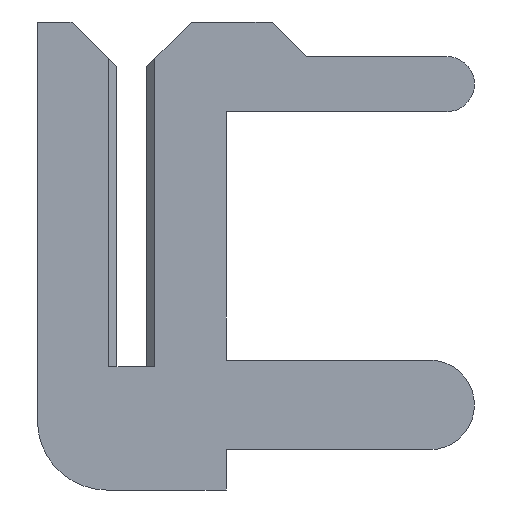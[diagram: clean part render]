
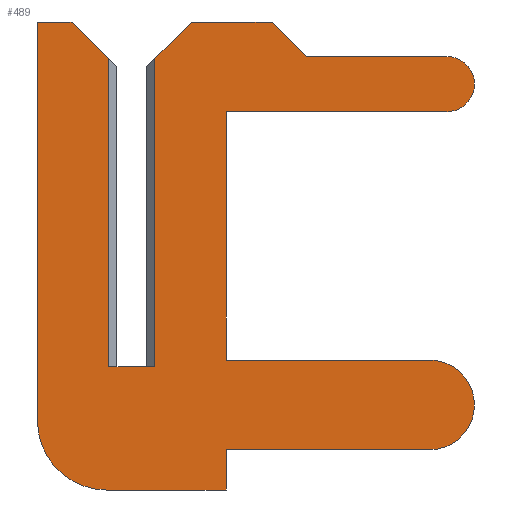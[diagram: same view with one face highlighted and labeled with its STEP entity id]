
A CAD part, left-side view. The second image highlights one B-rep face of the part: STEP entity #489.
In plain terms, the highlighted planar face has unit normal (-1, 0, 0).
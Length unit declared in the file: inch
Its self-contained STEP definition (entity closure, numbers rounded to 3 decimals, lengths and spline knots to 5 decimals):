
#2 = VECTOR ( 'NONE', #440, 39.37008 ) ;
#8 = CARTESIAN_POINT ( 'NONE',  ( -0.01, -0.1295, -0.036 ) ) ;
#13 = DIRECTION ( 'NONE',  ( 0., 0., 1. ) ) ;
#31 = CARTESIAN_POINT ( 'NONE',  ( -0.01, 0.0065, 0.1305 ) ) ;
#46 = ORIENTED_EDGE ( 'NONE', *, *, #446, .F. ) ;
#49 = VECTOR ( 'NONE', #506, 39.37008 ) ;
#58 = ORIENTED_EDGE ( 'NONE', *, *, #796, .F. ) ;
#72 = DIRECTION ( 'NONE',  ( -1., 0., 0. ) ) ;
#76 = CARTESIAN_POINT ( 'NONE',  ( -0.01, 0.01, 0. ) ) ;
#77 = VERTEX_POINT ( 'NONE', #879 ) ;
#81 = CARTESIAN_POINT ( 'NONE',  ( -0.01, -0.1295, 0.003 ) ) ;
#94 = VERTEX_POINT ( 'NONE', #270 ) ;
#100 = EDGE_CURVE ( 'NONE', #294, #377, #203, .T. ) ;
#101 = DIRECTION ( 'NONE',  ( 1., 0., 0. ) ) ;
#108 = CARTESIAN_POINT ( 'NONE',  ( -0.01, -0.041, -0.0535 ) ) ;
#149 = VERTEX_POINT ( 'NONE', #553 ) ;
#152 = DIRECTION ( 'NONE',  ( 0., 0., 1. ) ) ;
#155 = VERTEX_POINT ( 'NONE', #295 ) ;
#158 = CARTESIAN_POINT ( 'NONE',  ( -0.01, 0.011, -0.0535 ) ) ;
#161 = DIRECTION ( 'NONE',  ( 0., 0., 1. ) ) ;
#162 = VECTOR ( 'NONE', #549, 39.37008 ) ;
#163 = DIRECTION ( 'NONE',  ( 0., 1., 0. ) ) ;
#166 = CARTESIAN_POINT ( 'NONE',  ( -0.01, 0.011, -0.0235 ) ) ;
#179 = EDGE_CURVE ( 'NONE', #949, #963, #892, .T. ) ;
#185 = ORIENTED_EDGE ( 'NONE', *, *, #560, .F. ) ;
#188 = ORIENTED_EDGE ( 'NONE', *, *, #314, .F. ) ;
#200 = ORIENTED_EDGE ( 'NONE', *, *, #505, .F. ) ;
#203 = LINE ( 'NONE', #686, #2 ) ;
#206 = DIRECTION ( 'NONE',  ( 0., 0., 1. ) ) ;
#209 = LINE ( 'NONE', #882, #1025 ) ;
#211 = VERTEX_POINT ( 'NONE', #815 ) ;
#234 = ORIENTED_EDGE ( 'NONE', *, *, #867, .F. ) ;
#263 = VECTOR ( 'NONE', #206, 39.37008 ) ;
#266 = DIRECTION ( 'NONE',  ( 0., 0., -1. ) ) ;
#267 = ORIENTED_EDGE ( 'NONE', *, *, #837, .F. ) ;
#270 = CARTESIAN_POINT ( 'NONE',  ( -0.01, -0.137, 0.135 ) ) ;
#277 = DIRECTION ( 'NONE',  ( 0., -0.707, 0.707 ) ) ;
#287 = LINE ( 'NONE', #768, #49 ) ;
#294 = VERTEX_POINT ( 'NONE', #807 ) ;
#295 = CARTESIAN_POINT ( 'NONE',  ( -0.01, -0.076, 0.135 ) ) ;
#311 = CARTESIAN_POINT ( 'NONE',  ( -0.01, 0.011, -0.0235 ) ) ;
#314 = EDGE_CURVE ( 'NONE', #935, #493, #442, .T. ) ;
#323 = ORIENTED_EDGE ( 'NONE', *, *, #100, .F. ) ;
#326 = FACE_OUTER_BOUND ( 'NONE', #456, .T. ) ;
#333 = LINE ( 'NONE', #838, #644 ) ;
#340 = CARTESIAN_POINT ( 'NONE',  ( -0.01, -0.041, -0.036 ) ) ;
#345 = ORIENTED_EDGE ( 'NONE', *, *, #719, .F. ) ;
#362 = DIRECTION ( 'NONE',  ( 0., -1., 0. ) ) ;
#365 = CARTESIAN_POINT ( 'NONE',  ( -0.01, -0.041, -0.0535 ) ) ;
#367 = LINE ( 'NONE', #595, #394 ) ;
#377 = VERTEX_POINT ( 'NONE', #488 ) ;
#379 = LINE ( 'NONE', #31, #162 ) ;
#386 = ORIENTED_EDGE ( 'NONE', *, *, #917, .F. ) ;
#388 = EDGE_CURVE ( 'NONE', #493, #642, #333, .T. ) ;
#389 = LINE ( 'NONE', #845, #950 ) ;
#394 = VECTOR ( 'NONE', #869, 39.37008 ) ;
#407 = LINE ( 'NONE', #888, #263 ) ;
#410 = DIRECTION ( 'NONE',  ( 0., -1., 0. ) ) ;
#415 = VERTEX_POINT ( 'NONE', #654 ) ;
#422 = AXIS2_PLACEMENT_3D ( 'NONE', #166, #72, #161 ) ;
#428 = VECTOR ( 'NONE', #819, 39.37008 ) ;
#434 = LINE ( 'NONE', #969, #954 ) ;
#440 = DIRECTION ( 'NONE',  ( 0., -1., 0. ) ) ;
#442 = CIRCLE ( 'NONE', #554, 0.03 ) ;
#446 = EDGE_CURVE ( 'NONE', #415, #1122, #389, .T. ) ;
#456 = EDGE_LOOP ( 'NONE', ( #531, #806, #345, #1123, #234, #267, #778, #188, #185, #58, #967, #386, #46, #509, #200, #836, #615, #1089, #323 ) ) ;
#461 = CIRCLE ( 'NONE', #1072, 0.012 ) ;
#487 = VECTOR ( 'NONE', #981, 39.37008 ) ;
#488 = CARTESIAN_POINT ( 'NONE',  ( -0.01, -0.061, 0.15 ) ) ;
#489 = ADVANCED_FACE ( 'NONE', ( #326 ), #953, .T. ) ;
#493 = VERTEX_POINT ( 'NONE', #517 ) ;
#505 = EDGE_CURVE ( 'NONE', #906, #548, #287, .T. ) ;
#506 = DIRECTION ( 'NONE',  ( 0., 1., 0. ) ) ;
#509 = ORIENTED_EDGE ( 'NONE', *, *, #675, .F. ) ;
#517 = CARTESIAN_POINT ( 'NONE',  ( -0.01, 0.041, -0.0235 ) ) ;
#531 = ORIENTED_EDGE ( 'NONE', *, *, #756, .F. ) ;
#532 = VECTOR ( 'NONE', #362, 39.37008 ) ;
#542 = CARTESIAN_POINT ( 'NONE',  ( -0.01, 0.011, -0.0535 ) ) ;
#548 = VERTEX_POINT ( 'NONE', #673 ) ;
#549 = DIRECTION ( 'NONE',  ( 0., -0.707, -0.707 ) ) ;
#553 = CARTESIAN_POINT ( 'NONE',  ( -0.01, 0.026, 0.15 ) ) ;
#554 = AXIS2_PLACEMENT_3D ( 'NONE', #311, #578, #152 ) ;
#560 = EDGE_CURVE ( 'NONE', #864, #935, #769, .T. ) ;
#578 = DIRECTION ( 'NONE',  ( 1., 0., 0. ) ) ;
#595 = CARTESIAN_POINT ( 'NONE',  ( -0.01, -0.076, 0.135 ) ) ;
#597 = CARTESIAN_POINT ( 'NONE',  ( -0.01, -0.01, 0. ) ) ;
#604 = VERTEX_POINT ( 'NONE', #597 ) ;
#612 = CARTESIAN_POINT ( 'NONE',  ( -0.01, -0.137, 0.123 ) ) ;
#615 = ORIENTED_EDGE ( 'NONE', *, *, #929, .F. ) ;
#619 = VERTEX_POINT ( 'NONE', #76 ) ;
#634 = VECTOR ( 'NONE', #163, 39.37008 ) ;
#642 = VERTEX_POINT ( 'NONE', #705 ) ;
#644 = VECTOR ( 'NONE', #1108, 39.37008 ) ;
#654 = CARTESIAN_POINT ( 'NONE',  ( -0.01, -0.041, 0.003 ) ) ;
#673 = CARTESIAN_POINT ( 'NONE',  ( -0.01, -0.041, 0.111 ) ) ;
#675 = EDGE_CURVE ( 'NONE', #548, #415, #209, .T. ) ;
#682 = EDGE_CURVE ( 'NONE', #94, #906, #461, .T. ) ;
#686 = CARTESIAN_POINT ( 'NONE',  ( -0.01, -0.026, 0.15 ) ) ;
#687 = CARTESIAN_POINT ( 'NONE',  ( -0.01, -0.01, 0.15 ) ) ;
#688 = VECTOR ( 'NONE', #782, 39.37008 ) ;
#705 = CARTESIAN_POINT ( 'NONE',  ( -0.01, 0.041, 0.15 ) ) ;
#713 = DIRECTION ( 'NONE',  ( 1., 0., 0. ) ) ;
#719 = EDGE_CURVE ( 'NONE', #619, #604, #1125, .T. ) ;
#746 = LINE ( 'NONE', #365, #487 ) ;
#756 = EDGE_CURVE ( 'NONE', #77, #294, #434, .T. ) ;
#759 = VECTOR ( 'NONE', #266, 39.37008 ) ;
#768 = CARTESIAN_POINT ( 'NONE',  ( -0.01, -0.041, 0.111 ) ) ;
#769 = LINE ( 'NONE', #158, #634 ) ;
#776 = CARTESIAN_POINT ( 'NONE',  ( -0.01, 0.0065, 0. ) ) ;
#778 = ORIENTED_EDGE ( 'NONE', *, *, #388, .F. ) ;
#782 = DIRECTION ( 'NONE',  ( 0., -1., 0. ) ) ;
#793 = DIRECTION ( 'NONE',  ( 0., 0., -1. ) ) ;
#795 = LINE ( 'NONE', #1070, #885 ) ;
#796 = EDGE_CURVE ( 'NONE', #963, #864, #746, .T. ) ;
#802 = CARTESIAN_POINT ( 'NONE',  ( -0.01, -0.137, 0.111 ) ) ;
#806 = ORIENTED_EDGE ( 'NONE', *, *, #1018, .T. ) ;
#807 = CARTESIAN_POINT ( 'NONE',  ( -0.01, -0.026, 0.15 ) ) ;
#815 = CARTESIAN_POINT ( 'NONE',  ( -0.01, 0.01, 0.134 ) ) ;
#819 = DIRECTION ( 'NONE',  ( 0., 1., 0. ) ) ;
#836 = ORIENTED_EDGE ( 'NONE', *, *, #682, .F. ) ;
#837 = EDGE_CURVE ( 'NONE', #642, #149, #1054, .T. ) ;
#838 = CARTESIAN_POINT ( 'NONE',  ( -0.01, 0.041, 0.15 ) ) ;
#845 = CARTESIAN_POINT ( 'NONE',  ( -0.01, -0.1295, 0.003 ) ) ;
#853 = EDGE_CURVE ( 'NONE', #619, #211, #407, .T. ) ;
#864 = VERTEX_POINT ( 'NONE', #108 ) ;
#867 = EDGE_CURVE ( 'NONE', #149, #211, #379, .T. ) ;
#869 = DIRECTION ( 'NONE',  ( 0., -0.707, -0.707 ) ) ;
#879 = CARTESIAN_POINT ( 'NONE',  ( -0.01, -0.01, 0.134 ) ) ;
#882 = CARTESIAN_POINT ( 'NONE',  ( -0.01, -0.041, 0.003 ) ) ;
#885 = VECTOR ( 'NONE', #990, 39.37008 ) ;
#888 = CARTESIAN_POINT ( 'NONE',  ( -0.01, 0.01, -0.0235 ) ) ;
#892 = LINE ( 'NONE', #1099, #428 ) ;
#895 = CARTESIAN_POINT ( 'NONE',  ( -0.01, -0.1295, -0.0165 ) ) ;
#906 = VERTEX_POINT ( 'NONE', #802 ) ;
#911 = AXIS2_PLACEMENT_3D ( 'NONE', #895, #713, #983 ) ;
#917 = EDGE_CURVE ( 'NONE', #1122, #949, #1036, .T. ) ;
#929 = EDGE_CURVE ( 'NONE', #155, #94, #795, .T. ) ;
#935 = VERTEX_POINT ( 'NONE', #542 ) ;
#949 = VERTEX_POINT ( 'NONE', #8 ) ;
#950 = VECTOR ( 'NONE', #410, 39.37008 ) ;
#953 = PLANE ( 'NONE',  #422 ) ;
#954 = VECTOR ( 'NONE', #277, 39.37008 ) ;
#963 = VERTEX_POINT ( 'NONE', #340 ) ;
#967 = ORIENTED_EDGE ( 'NONE', *, *, #179, .F. ) ;
#969 = CARTESIAN_POINT ( 'NONE',  ( -0.01, -0.0065, 0.1305 ) ) ;
#981 = DIRECTION ( 'NONE',  ( 0., 0., -1. ) ) ;
#983 = DIRECTION ( 'NONE',  ( 0., 0., 1. ) ) ;
#990 = DIRECTION ( 'NONE',  ( 0., -1., 0. ) ) ;
#1018 = EDGE_CURVE ( 'NONE', #77, #604, #1113, .T. ) ;
#1025 = VECTOR ( 'NONE', #793, 39.37008 ) ;
#1036 = CIRCLE ( 'NONE', #911, 0.0195 ) ;
#1051 = CARTESIAN_POINT ( 'NONE',  ( -0.01, 0.026, 0.15 ) ) ;
#1054 = LINE ( 'NONE', #1051, #688 ) ;
#1070 = CARTESIAN_POINT ( 'NONE',  ( -0.01, -0.137, 0.135 ) ) ;
#1072 = AXIS2_PLACEMENT_3D ( 'NONE', #612, #101, #13 ) ;
#1079 = EDGE_CURVE ( 'NONE', #377, #155, #367, .T. ) ;
#1089 = ORIENTED_EDGE ( 'NONE', *, *, #1079, .F. ) ;
#1099 = CARTESIAN_POINT ( 'NONE',  ( -0.01, -0.041, -0.036 ) ) ;
#1108 = DIRECTION ( 'NONE',  ( 0., 0., 1. ) ) ;
#1113 = LINE ( 'NONE', #687, #759 ) ;
#1122 = VERTEX_POINT ( 'NONE', #81 ) ;
#1123 = ORIENTED_EDGE ( 'NONE', *, *, #853, .T. ) ;
#1125 = LINE ( 'NONE', #776, #532 ) ;
